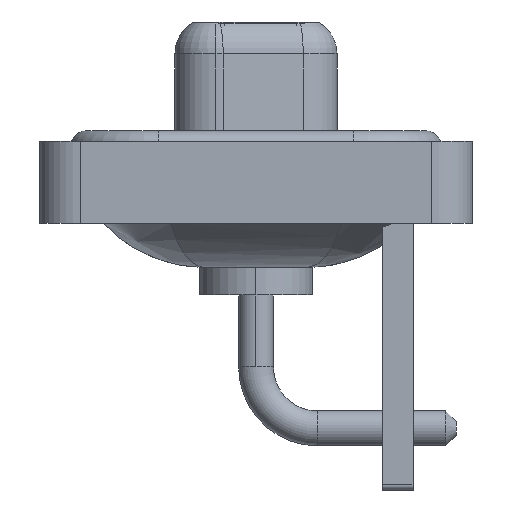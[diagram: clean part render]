
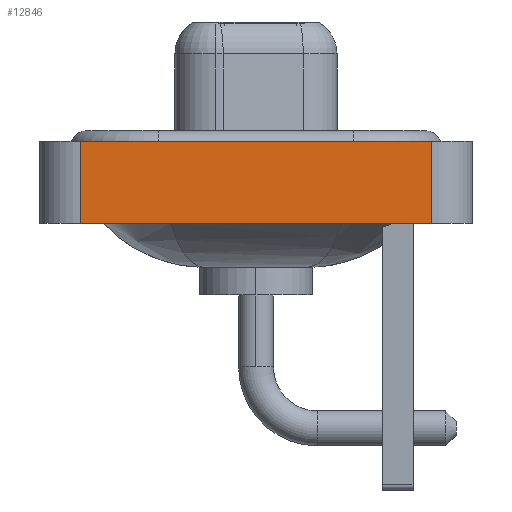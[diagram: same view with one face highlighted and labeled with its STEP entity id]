
A CAD part, left-side view. The second image highlights one B-rep face of the part: STEP entity #12846.
In plain terms, the highlighted planar face has unit normal (-1, 0, 0).
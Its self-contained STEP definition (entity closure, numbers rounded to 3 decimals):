
#519 = DIRECTION ( 'NONE',  ( 0., 0., 1. ) ) ;
#670 = EDGE_CURVE ( 'NONE', #6445, #6546, #13506, .T. ) ;
#974 = ORIENTED_EDGE ( 'NONE', *, *, #9677, .T. ) ;
#1794 = CARTESIAN_POINT ( 'NONE',  ( -7.3, 8.55, -3.6 ) ) ;
#2318 = AXIS2_PLACEMENT_3D ( 'NONE', #14635, #8111, #5722 ) ;
#4643 = DIRECTION ( 'NONE',  ( 0., 0., 1. ) ) ;
#4953 = LINE ( 'NONE', #10195, #14279 ) ;
#5722 = DIRECTION ( 'NONE',  ( 0., 0., 1. ) ) ;
#5791 = VERTEX_POINT ( 'NONE', #11803 ) ;
#6024 = EDGE_LOOP ( 'NONE', ( #974, #13614, #8693, #7368 ) ) ;
#6445 = VERTEX_POINT ( 'NONE', #14678 ) ;
#6546 = VERTEX_POINT ( 'NONE', #13462 ) ;
#6815 = CARTESIAN_POINT ( 'NONE',  ( -7.3, -8.55, 0.4 ) ) ;
#6838 = DIRECTION ( 'NONE',  ( 0., -1., 0. ) ) ;
#7368 = ORIENTED_EDGE ( 'NONE', *, *, #15344, .T. ) ;
#8111 = DIRECTION ( 'NONE',  ( -1., 0., 0. ) ) ;
#8296 = VERTEX_POINT ( 'NONE', #12962 ) ;
#8693 = ORIENTED_EDGE ( 'NONE', *, *, #670, .F. ) ;
#8881 = VECTOR ( 'NONE', #519, 1000. ) ;
#9329 = FACE_OUTER_BOUND ( 'NONE', #6024, .T. ) ;
#9429 = PLANE ( 'NONE',  #2318 ) ;
#9677 = EDGE_CURVE ( 'NONE', #5791, #8296, #12356, .T. ) ;
#10195 = CARTESIAN_POINT ( 'NONE',  ( -7.3, -8.55, -3.6 ) ) ;
#11803 = CARTESIAN_POINT ( 'NONE',  ( -7.3, -8.55, -3.6 ) ) ;
#11908 = EDGE_CURVE ( 'NONE', #6546, #8296, #15722, .T. ) ;
#12356 = LINE ( 'NONE', #16388, #15506 ) ;
#12641 = VECTOR ( 'NONE', #13151, 1000. ) ;
#12846 = ADVANCED_FACE ( 'NONE', ( #9329 ), #9429, .T. ) ;
#12962 = CARTESIAN_POINT ( 'NONE',  ( -7.3, -8.55, 0.4 ) ) ;
#13151 = DIRECTION ( 'NONE',  ( 0., -1., 0. ) ) ;
#13462 = CARTESIAN_POINT ( 'NONE',  ( -7.3, 8.55, 0.4 ) ) ;
#13506 = LINE ( 'NONE', #1794, #8881 ) ;
#13614 = ORIENTED_EDGE ( 'NONE', *, *, #11908, .F. ) ;
#14279 = VECTOR ( 'NONE', #6838, 1000. ) ;
#14635 = CARTESIAN_POINT ( 'NONE',  ( -7.3, -8.55, -3.6 ) ) ;
#14678 = CARTESIAN_POINT ( 'NONE',  ( -7.3, 8.55, -3.6 ) ) ;
#15344 = EDGE_CURVE ( 'NONE', #6445, #5791, #4953, .T. ) ;
#15506 = VECTOR ( 'NONE', #4643, 1000. ) ;
#15722 = LINE ( 'NONE', #6815, #12641 ) ;
#16388 = CARTESIAN_POINT ( 'NONE',  ( -7.3, -8.55, -3.6 ) ) ;
